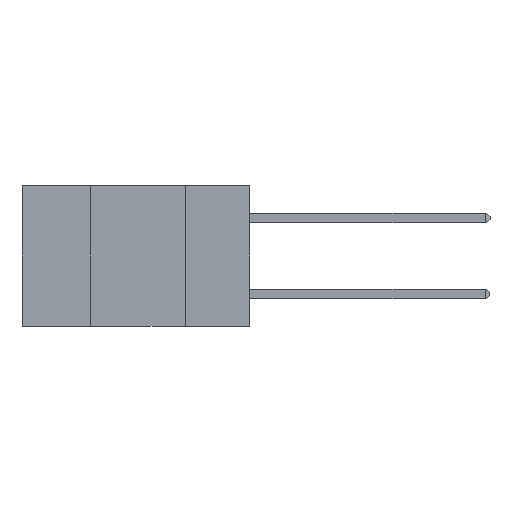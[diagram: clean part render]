
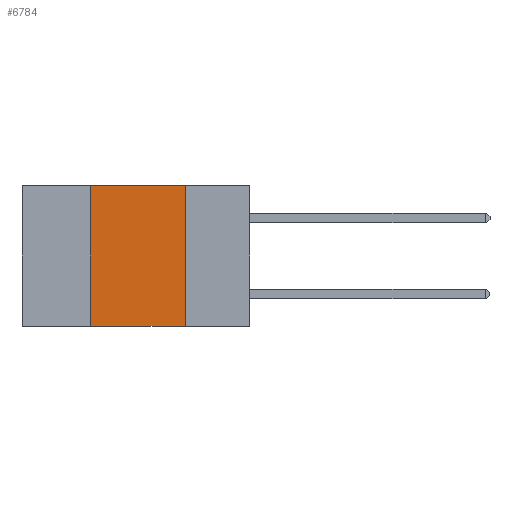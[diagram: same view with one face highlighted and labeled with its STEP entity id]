
A CAD part, left-side view. The second image highlights one B-rep face of the part: STEP entity #6784.
In plain terms, the highlighted planar face has unit normal (-1, 0, 0).
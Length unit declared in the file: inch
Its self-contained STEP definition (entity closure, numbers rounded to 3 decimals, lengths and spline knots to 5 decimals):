
#113 = LINE ( 'NONE', #3255, #6399 ) ;
#359 = EDGE_LOOP ( 'NONE', ( #13838, #8111, #6514, #6120 ) ) ;
#437 = DIRECTION ( 'NONE',  ( 0., 0., -1. ) ) ;
#884 = EDGE_CURVE ( 'NONE', #12545, #9834, #13145, .T. ) ;
#1284 = CARTESIAN_POINT ( 'NONE',  ( 0., 0.17, 0. ) ) ;
#1742 = CARTESIAN_POINT ( 'NONE',  ( 0., 0.6, 0. ) ) ;
#1863 = PLANE ( 'NONE',  #7659 ) ;
#2529 = CARTESIAN_POINT ( 'NONE',  ( 0., 0.42, -0.37 ) ) ;
#2658 = DIRECTION ( 'NONE',  ( 0., -1., 0. ) ) ;
#3255 = CARTESIAN_POINT ( 'NONE',  ( 0., 0.6, 0. ) ) ;
#3379 = LINE ( 'NONE', #11071, #6601 ) ;
#4124 = CARTESIAN_POINT ( 'NONE',  ( 0., 0.17, -0.37 ) ) ;
#4420 = VECTOR ( 'NONE', #11646, 39.37008 ) ;
#5099 = EDGE_CURVE ( 'NONE', #11866, #15520, #5428, .T. ) ;
#5428 = LINE ( 'NONE', #1284, #13763 ) ;
#6120 = ORIENTED_EDGE ( 'NONE', *, *, #14832, .T. ) ;
#6399 = VECTOR ( 'NONE', #12805, 39.37008 ) ;
#6514 = ORIENTED_EDGE ( 'NONE', *, *, #884, .F. ) ;
#6601 = VECTOR ( 'NONE', #2658, 39.37008 ) ;
#6784 = ADVANCED_FACE ( 'NONE', ( #8207 ), #1863, .F. ) ;
#7659 = AXIS2_PLACEMENT_3D ( 'NONE', #1742, #10929, #437 ) ;
#8111 = ORIENTED_EDGE ( 'NONE', *, *, #9611, .F. ) ;
#8207 = FACE_OUTER_BOUND ( 'NONE', #359, .T. ) ;
#9611 = EDGE_CURVE ( 'NONE', #9834, #11866, #113, .T. ) ;
#9744 = CARTESIAN_POINT ( 'NONE',  ( 0., 0.17, 0. ) ) ;
#9834 = VERTEX_POINT ( 'NONE', #13263 ) ;
#10696 = DIRECTION ( 'NONE',  ( 0., 0., -1. ) ) ;
#10929 = DIRECTION ( 'NONE',  ( 1., 0., 0. ) ) ;
#11071 = CARTESIAN_POINT ( 'NONE',  ( 0., 0.6, -0.37 ) ) ;
#11537 = CARTESIAN_POINT ( 'NONE',  ( 0., 0.42, 0. ) ) ;
#11646 = DIRECTION ( 'NONE',  ( 0., 0., 1. ) ) ;
#11866 = VERTEX_POINT ( 'NONE', #9744 ) ;
#12545 = VERTEX_POINT ( 'NONE', #2529 ) ;
#12805 = DIRECTION ( 'NONE',  ( 0., -1., 0. ) ) ;
#13145 = LINE ( 'NONE', #11537, #4420 ) ;
#13263 = CARTESIAN_POINT ( 'NONE',  ( 0., 0.42, 0. ) ) ;
#13763 = VECTOR ( 'NONE', #10696, 39.37008 ) ;
#13838 = ORIENTED_EDGE ( 'NONE', *, *, #5099, .F. ) ;
#14832 = EDGE_CURVE ( 'NONE', #12545, #15520, #3379, .T. ) ;
#15520 = VERTEX_POINT ( 'NONE', #4124 ) ;
